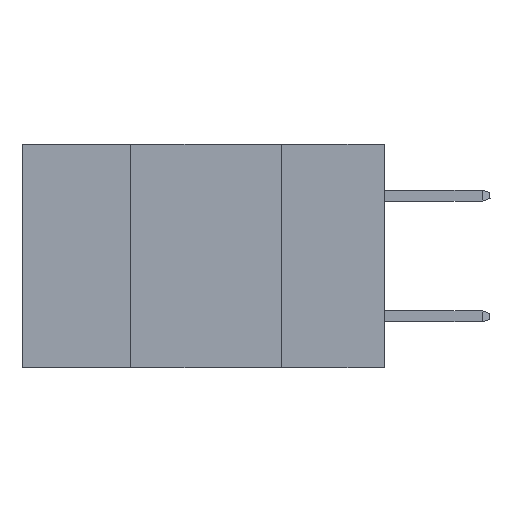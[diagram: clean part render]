
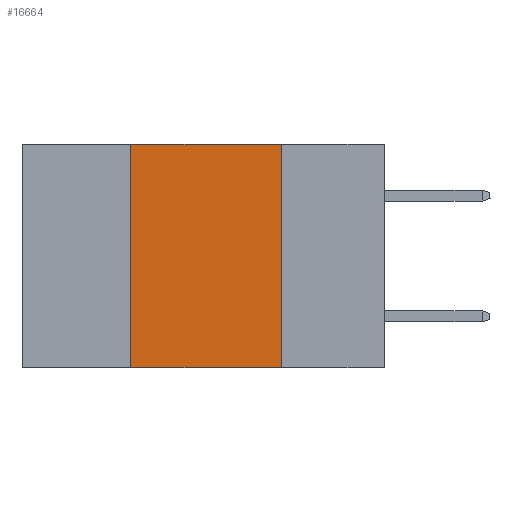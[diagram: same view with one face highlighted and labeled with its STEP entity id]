
A CAD part, left-side view. The second image highlights one B-rep face of the part: STEP entity #16664.
In plain terms, the highlighted planar face has unit normal (-1, 0, 0).
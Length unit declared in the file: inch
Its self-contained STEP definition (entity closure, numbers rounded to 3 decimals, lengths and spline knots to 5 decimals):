
#144 = EDGE_CURVE ( 'NONE', #2179, #12385, #2563, .T. ) ;
#428 = CARTESIAN_POINT ( 'NONE',  ( 0., 0.42, 0. ) ) ;
#742 = CARTESIAN_POINT ( 'NONE',  ( 0., 0.42, -0.37 ) ) ;
#748 = VECTOR ( 'NONE', #3597, 39.37008 ) ;
#920 = ORIENTED_EDGE ( 'NONE', *, *, #10003, .T. ) ;
#1091 = DIRECTION ( 'NONE',  ( 0., 0., 1. ) ) ;
#1100 = CARTESIAN_POINT ( 'NONE',  ( 0., 0.17, -0.37 ) ) ;
#1296 = LINE ( 'NONE', #13594, #7564 ) ;
#1969 = CARTESIAN_POINT ( 'NONE',  ( 0., 0.17, 0. ) ) ;
#2179 = VERTEX_POINT ( 'NONE', #1969 ) ;
#2202 = CARTESIAN_POINT ( 'NONE',  ( 0., 0.6, 0. ) ) ;
#2440 = LINE ( 'NONE', #9855, #4988 ) ;
#2563 = LINE ( 'NONE', #5014, #748 ) ;
#2888 = ORIENTED_EDGE ( 'NONE', *, *, #9332, .F. ) ;
#3597 = DIRECTION ( 'NONE',  ( 0., 0., -1. ) ) ;
#4123 = CARTESIAN_POINT ( 'NONE',  ( 0., 0.6, -0.37 ) ) ;
#4734 = DIRECTION ( 'NONE',  ( 0., -1., 0. ) ) ;
#4739 = FACE_OUTER_BOUND ( 'NONE', #13861, .T. ) ;
#4966 = LINE ( 'NONE', #4123, #17054 ) ;
#4988 = VECTOR ( 'NONE', #1091, 39.37008 ) ;
#5014 = CARTESIAN_POINT ( 'NONE',  ( 0., 0.17, 0. ) ) ;
#6451 = ORIENTED_EDGE ( 'NONE', *, *, #8988, .F. ) ;
#6631 = VERTEX_POINT ( 'NONE', #742 ) ;
#7564 = VECTOR ( 'NONE', #4734, 39.37008 ) ;
#8988 = EDGE_CURVE ( 'NONE', #16947, #2179, #1296, .T. ) ;
#9332 = EDGE_CURVE ( 'NONE', #6631, #16947, #2440, .T. ) ;
#9855 = CARTESIAN_POINT ( 'NONE',  ( 0., 0.42, 0. ) ) ;
#10003 = EDGE_CURVE ( 'NONE', #6631, #12385, #4966, .T. ) ;
#12385 = VERTEX_POINT ( 'NONE', #1100 ) ;
#13441 = ORIENTED_EDGE ( 'NONE', *, *, #144, .F. ) ;
#13469 = AXIS2_PLACEMENT_3D ( 'NONE', #2202, #18404, #17071 ) ;
#13594 = CARTESIAN_POINT ( 'NONE',  ( 0., 0.6, 0. ) ) ;
#13835 = PLANE ( 'NONE',  #13469 ) ;
#13861 = EDGE_LOOP ( 'NONE', ( #13441, #6451, #2888, #920 ) ) ;
#16664 = ADVANCED_FACE ( 'NONE', ( #4739 ), #13835, .F. ) ;
#16947 = VERTEX_POINT ( 'NONE', #428 ) ;
#17054 = VECTOR ( 'NONE', #18796, 39.37008 ) ;
#17071 = DIRECTION ( 'NONE',  ( 0., 0., -1. ) ) ;
#18404 = DIRECTION ( 'NONE',  ( 1., 0., 0. ) ) ;
#18796 = DIRECTION ( 'NONE',  ( 0., -1., 0. ) ) ;
